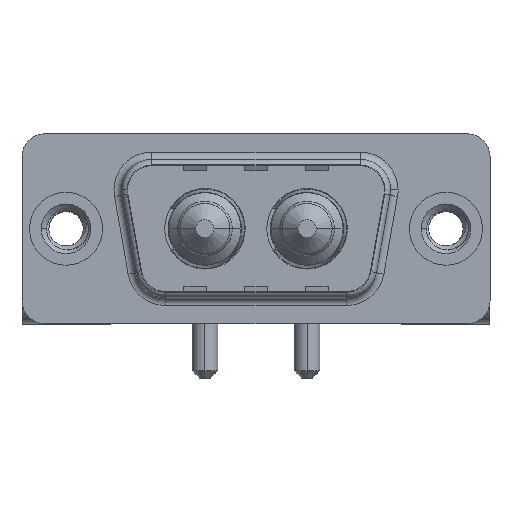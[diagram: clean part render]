
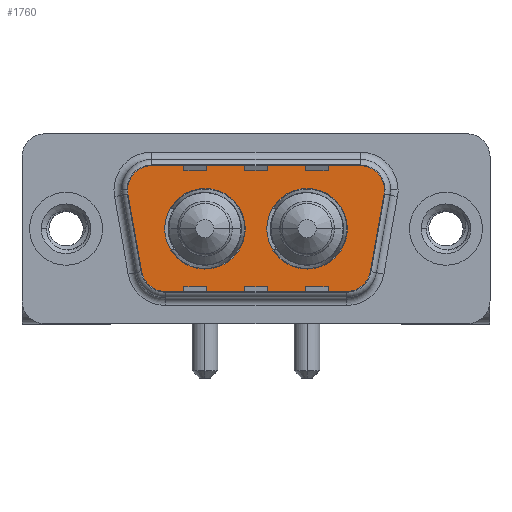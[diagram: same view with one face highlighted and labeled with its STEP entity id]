
A CAD part, top view. The second image highlights one B-rep face of the part: STEP entity #1760.
In plain terms, the highlighted planar face has unit normal (0, 0, 1).
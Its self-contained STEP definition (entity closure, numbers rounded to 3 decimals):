
#66 = DIRECTION ( 'NONE',  ( 0., 0., 1. ) ) ;
#420 = VECTOR ( 'NONE', #1320, 1000. ) ;
#456 = VERTEX_POINT ( 'NONE', #2603 ) ;
#663 = CARTESIAN_POINT ( 'NONE',  ( 18.541, -2.9, 0. ) ) ;
#758 = ORIENTED_EDGE ( 'NONE', *, *, #1684, .F. ) ;
#762 = VECTOR ( 'NONE', #10134, 1000. ) ;
#860 = CARTESIAN_POINT ( 'NONE',  ( 18.541, -4.9, 0. ) ) ;
#885 = VERTEX_POINT ( 'NONE', #4361 ) ;
#1126 = ORIENTED_EDGE ( 'NONE', *, *, #3902, .T. ) ;
#1293 = DIRECTION ( 'NONE',  ( 0.174, -0.985, 0. ) ) ;
#1320 = DIRECTION ( 'NONE',  ( 1., 0., 0. ) ) ;
#1491 = ORIENTED_EDGE ( 'NONE', *, *, #11202, .T. ) ;
#1519 = ORIENTED_EDGE ( 'NONE', *, *, #5141, .T. ) ;
#1633 = EDGE_CURVE ( 'NONE', #3787, #5021, #10273, .T. ) ;
#1643 = CARTESIAN_POINT ( 'NONE',  ( 6.459, -2.9, 0. ) ) ;
#1662 = ORIENTED_EDGE ( 'NONE', *, *, #2843, .F. ) ;
#1664 = VERTEX_POINT ( 'NONE', #9316 ) ;
#1684 = EDGE_CURVE ( 'NONE', #3057, #885, #5026, .T. ) ;
#1743 = AXIS2_PLACEMENT_3D ( 'NONE', #11902, #9938, #2396 ) ;
#1760 = ADVANCED_FACE ( 'NONE', ( #4444, #10457, #3486 ), #3672, .T. ) ;
#1822 = CIRCLE ( 'NONE', #9699, 2.65 ) ;
#1990 = EDGE_CURVE ( 'NONE', #8074, #9495, #5332, .T. ) ;
#2041 = CARTESIAN_POINT ( 'NONE',  ( 21.534, 2.553, 0. ) ) ;
#2152 = CARTESIAN_POINT ( 'NONE',  ( 9.14, 0., 0. ) ) ;
#2365 = VERTEX_POINT ( 'NONE', #7850 ) ;
#2396 = DIRECTION ( 'NONE',  ( 1., 0., 0. ) ) ;
#2498 = EDGE_CURVE ( 'NONE', #6995, #6604, #8026, .T. ) ;
#2527 = CARTESIAN_POINT ( 'NONE',  ( 5.436, 4.9, 0. ) ) ;
#2603 = CARTESIAN_POINT ( 'NONE',  ( 11.79, 0., 0. ) ) ;
#2698 = DIRECTION ( 'NONE',  ( 0., 0., 1. ) ) ;
#2707 = DIRECTION ( 'NONE',  ( 0., 0., 1. ) ) ;
#2800 = LINE ( 'NONE', #2041, #5230 ) ;
#2843 = EDGE_CURVE ( 'NONE', #456, #2947, #6792, .T. ) ;
#2947 = VERTEX_POINT ( 'NONE', #3328 ) ;
#3026 = CIRCLE ( 'NONE', #5048, 2.65 ) ;
#3030 = DIRECTION ( 'NONE',  ( 1., 0., 0. ) ) ;
#3057 = VERTEX_POINT ( 'NONE', #3635 ) ;
#3222 = CARTESIAN_POINT ( 'NONE',  ( 4.489, -3.247, 0. ) ) ;
#3328 = CARTESIAN_POINT ( 'NONE',  ( 6.49, 0., 0. ) ) ;
#3486 = FACE_OUTER_BOUND ( 'NONE', #6054, .T. ) ;
#3607 = DIRECTION ( 'NONE',  ( 1., 0., 0. ) ) ;
#3635 = CARTESIAN_POINT ( 'NONE',  ( 18.51, 0., 0. ) ) ;
#3672 = PLANE ( 'NONE',  #8911 ) ;
#3729 = CIRCLE ( 'NONE', #10623, 2. ) ;
#3784 = CIRCLE ( 'NONE', #7043, 2. ) ;
#3787 = VERTEX_POINT ( 'NONE', #10961 ) ;
#3902 = EDGE_CURVE ( 'NONE', #9495, #1664, #3729, .T. ) ;
#4006 = EDGE_LOOP ( 'NONE', ( #758, #7317 ) ) ;
#4361 = CARTESIAN_POINT ( 'NONE',  ( 13.21, 0., 0. ) ) ;
#4444 = FACE_BOUND ( 'NONE', #4006, .T. ) ;
#4535 = DIRECTION ( 'NONE',  ( 0., 0., 1. ) ) ;
#4633 = DIRECTION ( 'NONE',  ( 1., 0., 0. ) ) ;
#4692 = CARTESIAN_POINT ( 'NONE',  ( 19.564, 2.9, 0. ) ) ;
#4870 = DIRECTION ( 'NONE',  ( 0., 0., 1. ) ) ;
#4910 = ORIENTED_EDGE ( 'NONE', *, *, #8057, .T. ) ;
#5021 = VERTEX_POINT ( 'NONE', #12485 ) ;
#5026 = CIRCLE ( 'NONE', #11486, 2.65 ) ;
#5048 = AXIS2_PLACEMENT_3D ( 'NONE', #7094, #4870, #3030 ) ;
#5063 = EDGE_LOOP ( 'NONE', ( #1662, #8242 ) ) ;
#5141 = EDGE_CURVE ( 'NONE', #2365, #7033, #5330, .T. ) ;
#5230 = VECTOR ( 'NONE', #11601, 1000. ) ;
#5330 = LINE ( 'NONE', #2527, #762 ) ;
#5332 = LINE ( 'NONE', #10968, #7306 ) ;
#5583 = AXIS2_PLACEMENT_3D ( 'NONE', #2152, #9120, #11084 ) ;
#5615 = DIRECTION ( 'NONE',  ( -1., 0., 0. ) ) ;
#5617 = ORIENTED_EDGE ( 'NONE', *, *, #11855, .T. ) ;
#5625 = DIRECTION ( 'NONE',  ( -1., 0., 0. ) ) ;
#5647 = DIRECTION ( 'NONE',  ( -1., 0., 0. ) ) ;
#5697 = DIRECTION ( 'NONE',  ( 1., 0., 0. ) ) ;
#5730 = EDGE_CURVE ( 'NONE', #5021, #2365, #3784, .T. ) ;
#5797 = DIRECTION ( 'NONE',  ( 1., 0., 0. ) ) ;
#6054 = EDGE_LOOP ( 'NONE', ( #10339, #4910, #6173, #6324, #1519, #1491, #6380, #1126, #5617 ) ) ;
#6173 = ORIENTED_EDGE ( 'NONE', *, *, #1633, .T. ) ;
#6324 = ORIENTED_EDGE ( 'NONE', *, *, #5730, .T. ) ;
#6380 = ORIENTED_EDGE ( 'NONE', *, *, #1990, .T. ) ;
#6604 = VERTEX_POINT ( 'NONE', #7827 ) ;
#6792 = CIRCLE ( 'NONE', #5583, 2.65 ) ;
#6995 = VERTEX_POINT ( 'NONE', #860 ) ;
#7033 = VERTEX_POINT ( 'NONE', #8562 ) ;
#7043 = AXIS2_PLACEMENT_3D ( 'NONE', #12445, #4535, #5615 ) ;
#7094 = CARTESIAN_POINT ( 'NONE',  ( 9.14, 0., 0. ) ) ;
#7306 = VECTOR ( 'NONE', #1293, 1000. ) ;
#7317 = ORIENTED_EDGE ( 'NONE', *, *, #10677, .F. ) ;
#7581 = CARTESIAN_POINT ( 'NONE',  ( 5.436, 2.9, 0. ) ) ;
#7827 = CARTESIAN_POINT ( 'NONE',  ( 20.511, -3.247, 0. ) ) ;
#7850 = CARTESIAN_POINT ( 'NONE',  ( 19.564, 4.9, 0. ) ) ;
#8026 = CIRCLE ( 'NONE', #1743, 2. ) ;
#8057 = EDGE_CURVE ( 'NONE', #6604, #3787, #2800, .T. ) ;
#8074 = VERTEX_POINT ( 'NONE', #10529 ) ;
#8151 = CARTESIAN_POINT ( 'NONE',  ( 6.459, -4.9, 0. ) ) ;
#8242 = ORIENTED_EDGE ( 'NONE', *, *, #9506, .F. ) ;
#8552 = CARTESIAN_POINT ( 'NONE',  ( 15.86, 0., 0. ) ) ;
#8562 = CARTESIAN_POINT ( 'NONE',  ( 5.436, 4.9, 0. ) ) ;
#8911 = AXIS2_PLACEMENT_3D ( 'NONE', #663, #11282, #4633 ) ;
#9120 = DIRECTION ( 'NONE',  ( 0., 0., 1. ) ) ;
#9278 = CIRCLE ( 'NONE', #12318, 2. ) ;
#9316 = CARTESIAN_POINT ( 'NONE',  ( 6.459, -4.9, 0. ) ) ;
#9373 = DIRECTION ( 'NONE',  ( 0., 0., 1. ) ) ;
#9488 = CARTESIAN_POINT ( 'NONE',  ( 15.86, 0., 0. ) ) ;
#9495 = VERTEX_POINT ( 'NONE', #3222 ) ;
#9506 = EDGE_CURVE ( 'NONE', #2947, #456, #3026, .T. ) ;
#9699 = AXIS2_PLACEMENT_3D ( 'NONE', #9488, #66, #5697 ) ;
#9938 = DIRECTION ( 'NONE',  ( 0., 0., 1. ) ) ;
#10080 = AXIS2_PLACEMENT_3D ( 'NONE', #4692, #9373, #5647 ) ;
#10134 = DIRECTION ( 'NONE',  ( -1., 0., 0. ) ) ;
#10273 = CIRCLE ( 'NONE', #10080, 2. ) ;
#10339 = ORIENTED_EDGE ( 'NONE', *, *, #2498, .T. ) ;
#10457 = FACE_BOUND ( 'NONE', #5063, .T. ) ;
#10529 = CARTESIAN_POINT ( 'NONE',  ( 3.466, 2.553, 0. ) ) ;
#10623 = AXIS2_PLACEMENT_3D ( 'NONE', #1643, #2707, #5625 ) ;
#10677 = EDGE_CURVE ( 'NONE', #885, #3057, #1822, .T. ) ;
#10961 = CARTESIAN_POINT ( 'NONE',  ( 21.534, 2.553, 0. ) ) ;
#10968 = CARTESIAN_POINT ( 'NONE',  ( 3.466, 2.553, 0. ) ) ;
#11084 = DIRECTION ( 'NONE',  ( 1., 0., 0. ) ) ;
#11202 = EDGE_CURVE ( 'NONE', #7033, #8074, #9278, .T. ) ;
#11282 = DIRECTION ( 'NONE',  ( 0., 0., 1. ) ) ;
#11486 = AXIS2_PLACEMENT_3D ( 'NONE', #8552, #12288, #3607 ) ;
#11601 = DIRECTION ( 'NONE',  ( 0.174, 0.985, 0. ) ) ;
#11855 = EDGE_CURVE ( 'NONE', #1664, #6995, #12006, .T. ) ;
#11902 = CARTESIAN_POINT ( 'NONE',  ( 18.541, -2.9, 0. ) ) ;
#12006 = LINE ( 'NONE', #8151, #420 ) ;
#12288 = DIRECTION ( 'NONE',  ( 0., 0., 1. ) ) ;
#12318 = AXIS2_PLACEMENT_3D ( 'NONE', #7581, #2698, #5797 ) ;
#12445 = CARTESIAN_POINT ( 'NONE',  ( 19.564, 2.9, 0. ) ) ;
#12485 = CARTESIAN_POINT ( 'NONE',  ( 21.564, 2.9, 0. ) ) ;
